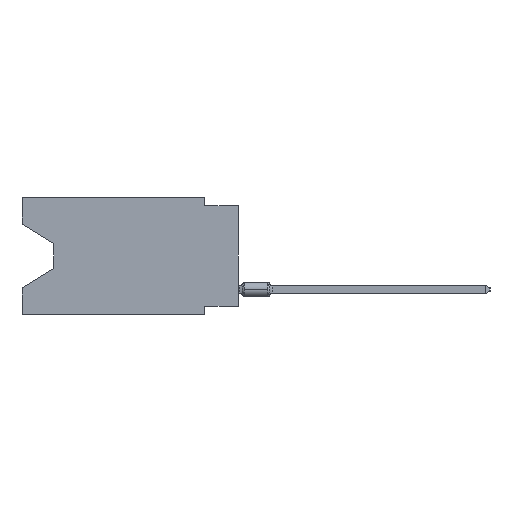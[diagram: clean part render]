
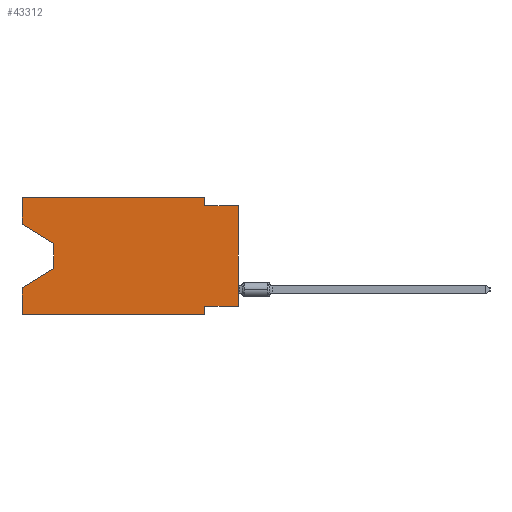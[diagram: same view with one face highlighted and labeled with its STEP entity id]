
A CAD part, left-side view. The second image highlights one B-rep face of the part: STEP entity #43312.
In plain terms, the highlighted planar face has unit normal (-1, 0, 0).
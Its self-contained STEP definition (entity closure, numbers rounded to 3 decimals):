
#3508 = ORIENTED_EDGE ( 'NONE', *, *, #28843, .T. ) ;
#3663 = CARTESIAN_POINT ( 'NONE',  ( 0., 0., -8.255 ) ) ;
#4043 = VECTOR ( 'NONE', #86214, 1000. ) ;
#5020 = CARTESIAN_POINT ( 'NONE',  ( 0., 16.383, 0. ) ) ;
#5088 = EDGE_CURVE ( 'NONE', #49363, #33263, #97348, .T. ) ;
#6668 = CARTESIAN_POINT ( 'NONE',  ( 0., 0., -0.635 ) ) ;
#8133 = EDGE_CURVE ( 'NONE', #49833, #17922, #66384, .T. ) ;
#9054 = ORIENTED_EDGE ( 'NONE', *, *, #5088, .F. ) ;
#9354 = LINE ( 'NONE', #72552, #113867 ) ;
#11778 = CARTESIAN_POINT ( 'NONE',  ( 0., 13.97, -3.505 ) ) ;
#12591 = LINE ( 'NONE', #3663, #21308 ) ;
#13325 = VECTOR ( 'NONE', #76935, 1000. ) ;
#13381 = FACE_OUTER_BOUND ( 'NONE', #58008, .T. ) ;
#13797 = VERTEX_POINT ( 'NONE', #51989 ) ;
#13798 = CARTESIAN_POINT ( 'NONE',  ( 0., 16.383, -2.038 ) ) ;
#16155 = ORIENTED_EDGE ( 'NONE', *, *, #24969, .F. ) ;
#16599 = CARTESIAN_POINT ( 'NONE',  ( 0., 16.383, -6.852 ) ) ;
#17922 = VERTEX_POINT ( 'NONE', #11778 ) ;
#20921 = VERTEX_POINT ( 'NONE', #34404 ) ;
#21105 = LINE ( 'NONE', #50882, #76715 ) ;
#21308 = VECTOR ( 'NONE', #59051, 1000. ) ;
#23489 = CARTESIAN_POINT ( 'NONE',  ( 0., 16.383, -8.89 ) ) ;
#23528 = PLANE ( 'NONE',  #101954 ) ;
#23576 = ORIENTED_EDGE ( 'NONE', *, *, #32465, .T. ) ;
#24969 = EDGE_CURVE ( 'NONE', #116860, #20921, #70433, .T. ) ;
#26847 = VECTOR ( 'NONE', #45507, 1000. ) ;
#28843 = EDGE_CURVE ( 'NONE', #49363, #64770, #9354, .T. ) ;
#32465 = EDGE_CURVE ( 'NONE', #52464, #33263, #107219, .T. ) ;
#33263 = VERTEX_POINT ( 'NONE', #16599 ) ;
#33580 = CARTESIAN_POINT ( 'NONE',  ( 0., 16.383, 0. ) ) ;
#34404 = CARTESIAN_POINT ( 'NONE',  ( 0., 0., -0.635 ) ) ;
#36673 = ORIENTED_EDGE ( 'NONE', *, *, #90740, .F. ) ;
#40576 = CARTESIAN_POINT ( 'NONE',  ( 0., 2.54, 0. ) ) ;
#40717 = VECTOR ( 'NONE', #43024, 1000. ) ;
#42586 = DIRECTION ( 'NONE',  ( 1., 0., 0. ) ) ;
#43024 = DIRECTION ( 'NONE',  ( 0., -1., 0. ) ) ;
#43312 = ADVANCED_FACE ( 'NONE', ( #13381 ), #23528, .F. ) ;
#45507 = DIRECTION ( 'NONE',  ( 0., 0., -1. ) ) ;
#45849 = VECTOR ( 'NONE', #79840, 1000. ) ;
#49154 = CARTESIAN_POINT ( 'NONE',  ( 0., 16.383, 0. ) ) ;
#49363 = VERTEX_POINT ( 'NONE', #23489 ) ;
#49833 = VERTEX_POINT ( 'NONE', #13798 ) ;
#50882 = CARTESIAN_POINT ( 'NONE',  ( 0., 16.383, 0. ) ) ;
#51784 = ORIENTED_EDGE ( 'NONE', *, *, #91430, .F. ) ;
#51989 = CARTESIAN_POINT ( 'NONE',  ( 0., 0., -8.255 ) ) ;
#52464 = VERTEX_POINT ( 'NONE', #91030 ) ;
#53366 = VERTEX_POINT ( 'NONE', #105390 ) ;
#58008 = EDGE_LOOP ( 'NONE', ( #112058, #60107, #23576, #9054, #3508, #79267, #36673, #83125, #16155, #91227, #85626, #51784 ) ) ;
#59051 = DIRECTION ( 'NONE',  ( 0., 1., 0. ) ) ;
#59134 = VERTEX_POINT ( 'NONE', #109938 ) ;
#60008 = CARTESIAN_POINT ( 'NONE',  ( 0., 16.383, 0. ) ) ;
#60107 = ORIENTED_EDGE ( 'NONE', *, *, #96487, .T. ) ;
#62401 = VECTOR ( 'NONE', #102135, 1000. ) ;
#62774 = LINE ( 'NONE', #71731, #26847 ) ;
#63968 = EDGE_CURVE ( 'NONE', #13797, #20921, #78467, .T. ) ;
#64494 = EDGE_CURVE ( 'NONE', #66789, #59134, #106252, .T. ) ;
#64770 = VERTEX_POINT ( 'NONE', #74622 ) ;
#66384 = LINE ( 'NONE', #76523, #62401 ) ;
#66789 = VERTEX_POINT ( 'NONE', #60008 ) ;
#68857 = CARTESIAN_POINT ( 'NONE',  ( 0., 13.97, -3.505 ) ) ;
#69632 = VECTOR ( 'NONE', #105177, 1000. ) ;
#70433 = LINE ( 'NONE', #6668, #40717 ) ;
#70525 = DIRECTION ( 'NONE',  ( 0., -1., 0. ) ) ;
#71731 = CARTESIAN_POINT ( 'NONE',  ( 0., 2.54, -8.89 ) ) ;
#72552 = CARTESIAN_POINT ( 'NONE',  ( 0., 16.383, -8.89 ) ) ;
#73597 = CARTESIAN_POINT ( 'NONE',  ( 0., 2.54, -0.635 ) ) ;
#74622 = CARTESIAN_POINT ( 'NONE',  ( 0., 2.54, -8.89 ) ) ;
#76523 = CARTESIAN_POINT ( 'NONE',  ( 0., 16.383, -2.038 ) ) ;
#76676 = EDGE_CURVE ( 'NONE', #59134, #116860, #85833, .T. ) ;
#76715 = VECTOR ( 'NONE', #93794, 1000. ) ;
#76935 = DIRECTION ( 'NONE',  ( 0., 0., -1. ) ) ;
#78339 = DIRECTION ( 'NONE',  ( 0., 0., -1. ) ) ;
#78467 = LINE ( 'NONE', #104063, #4043 ) ;
#79267 = ORIENTED_EDGE ( 'NONE', *, *, #102713, .F. ) ;
#79840 = DIRECTION ( 'NONE',  ( 0., 0.855, -0.519 ) ) ;
#83125 = ORIENTED_EDGE ( 'NONE', *, *, #63968, .T. ) ;
#85626 = ORIENTED_EDGE ( 'NONE', *, *, #64494, .F. ) ;
#85833 = LINE ( 'NONE', #40576, #13325 ) ;
#86214 = DIRECTION ( 'NONE',  ( 0., 0., 1. ) ) ;
#90740 = EDGE_CURVE ( 'NONE', #13797, #53366, #12591, .T. ) ;
#91030 = CARTESIAN_POINT ( 'NONE',  ( 0., 13.97, -5.385 ) ) ;
#91227 = ORIENTED_EDGE ( 'NONE', *, *, #76676, .F. ) ;
#91430 = EDGE_CURVE ( 'NONE', #49833, #66789, #21105, .T. ) ;
#93794 = DIRECTION ( 'NONE',  ( 0., 0., 1. ) ) ;
#96487 = EDGE_CURVE ( 'NONE', #17922, #52464, #112322, .T. ) ;
#97348 = LINE ( 'NONE', #5020, #99844 ) ;
#99844 = VECTOR ( 'NONE', #106856, 1000. ) ;
#101954 = AXIS2_PLACEMENT_3D ( 'NONE', #49154, #42586, #78339 ) ;
#102135 = DIRECTION ( 'NONE',  ( 0., -0.855, -0.519 ) ) ;
#102713 = EDGE_CURVE ( 'NONE', #53366, #64770, #62774, .T. ) ;
#104063 = CARTESIAN_POINT ( 'NONE',  ( 0., 0., 0. ) ) ;
#105177 = DIRECTION ( 'NONE',  ( 0., 0., -1. ) ) ;
#105390 = CARTESIAN_POINT ( 'NONE',  ( 0., 2.54, -8.255 ) ) ;
#106252 = LINE ( 'NONE', #33580, #108729 ) ;
#106856 = DIRECTION ( 'NONE',  ( 0., 0., 1. ) ) ;
#107219 = LINE ( 'NONE', #116747, #45849 ) ;
#108729 = VECTOR ( 'NONE', #70525, 1000. ) ;
#109452 = DIRECTION ( 'NONE',  ( 0., -1., 0. ) ) ;
#109938 = CARTESIAN_POINT ( 'NONE',  ( 0., 2.54, 0. ) ) ;
#112058 = ORIENTED_EDGE ( 'NONE', *, *, #8133, .T. ) ;
#112322 = LINE ( 'NONE', #68857, #69632 ) ;
#113867 = VECTOR ( 'NONE', #109452, 1000. ) ;
#116747 = CARTESIAN_POINT ( 'NONE',  ( 0., 13.97, -5.385 ) ) ;
#116860 = VERTEX_POINT ( 'NONE', #73597 ) ;
